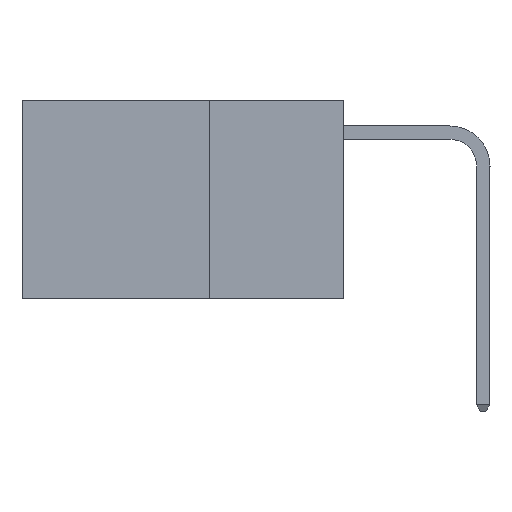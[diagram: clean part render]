
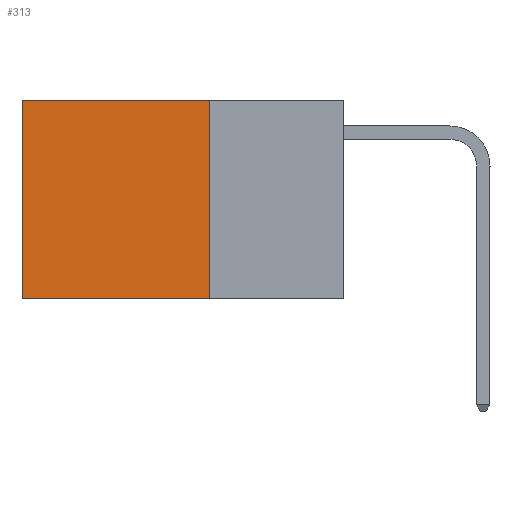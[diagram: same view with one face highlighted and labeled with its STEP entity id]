
A CAD part, left-side view. The second image highlights one B-rep face of the part: STEP entity #313.
In plain terms, the highlighted planar face has unit normal (-1, 0, 0).
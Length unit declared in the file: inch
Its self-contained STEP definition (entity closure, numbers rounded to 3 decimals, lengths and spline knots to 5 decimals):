
#281 = ORIENTED_EDGE ( 'NONE', *, *, #6490, .T. ) ;
#313 = ADVANCED_FACE ( 'NONE', ( #14707 ), #22088, .F. ) ;
#924 = CARTESIAN_POINT ( 'NONE',  ( 0.2625, 0.25, -0.37 ) ) ;
#1890 = VERTEX_POINT ( 'NONE', #18345 ) ;
#4388 = CARTESIAN_POINT ( 'NONE',  ( 0.2625, 0.25, 0. ) ) ;
#4768 = DIRECTION ( 'NONE',  ( 0., 0., -1. ) ) ;
#6490 = EDGE_CURVE ( 'NONE', #28548, #10515, #24097, .T. ) ;
#6842 = EDGE_CURVE ( 'NONE', #18375, #1890, #20821, .T. ) ;
#7578 = VECTOR ( 'NONE', #7792, 39.37008 ) ;
#7630 = VECTOR ( 'NONE', #22038, 39.37008 ) ;
#7698 = LINE ( 'NONE', #9393, #25580 ) ;
#7792 = DIRECTION ( 'NONE',  ( 0., 0., -1. ) ) ;
#9393 = CARTESIAN_POINT ( 'NONE',  ( 0.2625, 0.25, 0. ) ) ;
#10456 = DIRECTION ( 'NONE',  ( 0., 0., -1. ) ) ;
#10515 = VERTEX_POINT ( 'NONE', #13475 ) ;
#12668 = AXIS2_PLACEMENT_3D ( 'NONE', #24319, #24424, #10456 ) ;
#13475 = CARTESIAN_POINT ( 'NONE',  ( 0.2625, 0.6, 0. ) ) ;
#13805 = DIRECTION ( 'NONE',  ( 0., 1., 0. ) ) ;
#14526 = EDGE_CURVE ( 'NONE', #10515, #1890, #20028, .T. ) ;
#14707 = FACE_OUTER_BOUND ( 'NONE', #23644, .T. ) ;
#15197 = ORIENTED_EDGE ( 'NONE', *, *, #6842, .F. ) ;
#17906 = VECTOR ( 'NONE', #13805, 39.37008 ) ;
#18153 = CARTESIAN_POINT ( 'NONE',  ( 0.2625, 0.25, 0. ) ) ;
#18345 = CARTESIAN_POINT ( 'NONE',  ( 0.2625, 0.6, -0.37 ) ) ;
#18375 = VERTEX_POINT ( 'NONE', #924 ) ;
#19486 = CARTESIAN_POINT ( 'NONE',  ( 0.2625, 0.6, 0. ) ) ;
#19700 = ORIENTED_EDGE ( 'NONE', *, *, #14526, .T. ) ;
#20028 = LINE ( 'NONE', #19486, #7578 ) ;
#20821 = LINE ( 'NONE', #26577, #7630 ) ;
#22038 = DIRECTION ( 'NONE',  ( 0., 1., 0. ) ) ;
#22088 = PLANE ( 'NONE',  #12668 ) ;
#23644 = EDGE_LOOP ( 'NONE', ( #19700, #15197, #25161, #281 ) ) ;
#24097 = LINE ( 'NONE', #4388, #17906 ) ;
#24319 = CARTESIAN_POINT ( 'NONE',  ( 0.2625, 0.25, 0. ) ) ;
#24424 = DIRECTION ( 'NONE',  ( 1., 0., 0. ) ) ;
#25161 = ORIENTED_EDGE ( 'NONE', *, *, #27839, .F. ) ;
#25580 = VECTOR ( 'NONE', #4768, 39.37008 ) ;
#26577 = CARTESIAN_POINT ( 'NONE',  ( 0.2625, 0.25, -0.37 ) ) ;
#27839 = EDGE_CURVE ( 'NONE', #28548, #18375, #7698, .T. ) ;
#28548 = VERTEX_POINT ( 'NONE', #18153 ) ;
